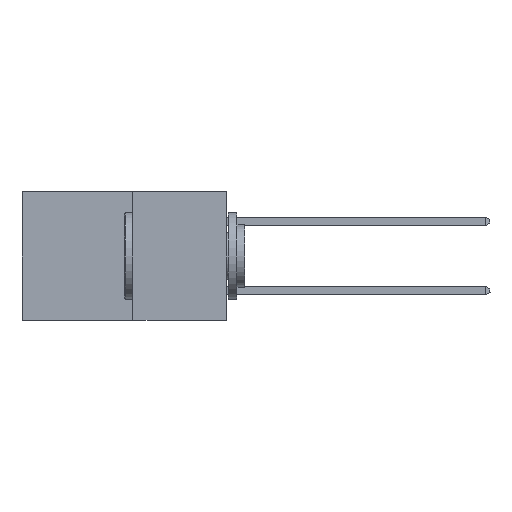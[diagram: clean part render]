
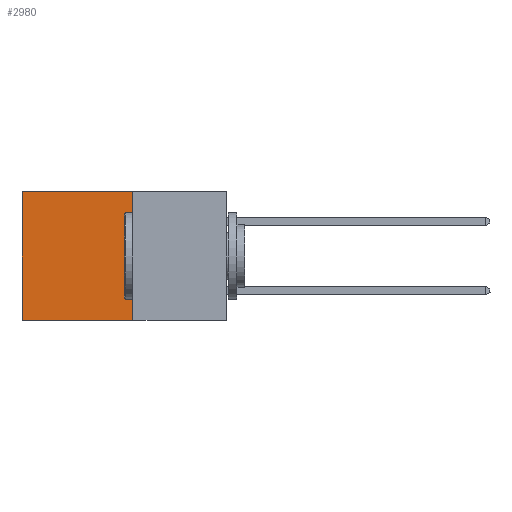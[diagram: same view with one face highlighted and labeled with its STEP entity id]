
A CAD part, left-side view. The second image highlights one B-rep face of the part: STEP entity #2980.
In plain terms, the highlighted planar face has unit normal (-1, 0, 0).
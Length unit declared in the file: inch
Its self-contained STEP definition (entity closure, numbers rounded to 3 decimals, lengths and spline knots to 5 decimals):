
#1551 = LINE ( 'NONE', #14602, #8207 ) ;
#2940 = VECTOR ( 'NONE', #19066, 39.37008 ) ;
#2980 = ADVANCED_FACE ( 'NONE', ( #14730 ), #12413, .F. ) ;
#3741 = EDGE_LOOP ( 'NONE', ( #17220, #11956, #30490, #20516 ) ) ;
#6551 = CARTESIAN_POINT ( 'NONE',  ( 0.277, 0.59, -0.37 ) ) ;
#8207 = VECTOR ( 'NONE', #31452, 39.37008 ) ;
#8642 = CARTESIAN_POINT ( 'NONE',  ( 0.277, 0.27, -0.37 ) ) ;
#9600 = LINE ( 'NONE', #11668, #2940 ) ;
#10718 = VECTOR ( 'NONE', #21757, 39.37008 ) ;
#11668 = CARTESIAN_POINT ( 'NONE',  ( 0.277, 0.27, -0.37 ) ) ;
#11956 = ORIENTED_EDGE ( 'NONE', *, *, #24869, .F. ) ;
#12086 = DIRECTION ( 'NONE',  ( 0., 0., -1. ) ) ;
#12127 = DIRECTION ( 'NONE',  ( 1., 0., 0. ) ) ;
#12413 = PLANE ( 'NONE',  #14323 ) ;
#12559 = CARTESIAN_POINT ( 'NONE',  ( 0.277, 0.27, -0.37 ) ) ;
#13014 = VERTEX_POINT ( 'NONE', #8642 ) ;
#13488 = VECTOR ( 'NONE', #16555, 39.37008 ) ;
#14093 = CARTESIAN_POINT ( 'NONE',  ( 0.277, 0.59, -0.37 ) ) ;
#14323 = AXIS2_PLACEMENT_3D ( 'NONE', #12559, #12127, #12086 ) ;
#14602 = CARTESIAN_POINT ( 'NONE',  ( 0.277, 0.27, 0. ) ) ;
#14627 = EDGE_CURVE ( 'NONE', #21737, #13014, #23674, .T. ) ;
#14730 = FACE_OUTER_BOUND ( 'NONE', #3741, .T. ) ;
#16555 = DIRECTION ( 'NONE',  ( 0., 0., -1. ) ) ;
#17220 = ORIENTED_EDGE ( 'NONE', *, *, #23754, .T. ) ;
#17241 = EDGE_CURVE ( 'NONE', #21737, #30504, #1551, .T. ) ;
#18993 = CARTESIAN_POINT ( 'NONE',  ( 0.277, 0.27, 0. ) ) ;
#19066 = DIRECTION ( 'NONE',  ( 0., 1., 0. ) ) ;
#19327 = CARTESIAN_POINT ( 'NONE',  ( 0.277, 0.27, -0.37 ) ) ;
#19961 = LINE ( 'NONE', #14093, #13488 ) ;
#20516 = ORIENTED_EDGE ( 'NONE', *, *, #17241, .T. ) ;
#20989 = VERTEX_POINT ( 'NONE', #6551 ) ;
#21737 = VERTEX_POINT ( 'NONE', #18993 ) ;
#21757 = DIRECTION ( 'NONE',  ( 0., 0., -1. ) ) ;
#23674 = LINE ( 'NONE', #19327, #10718 ) ;
#23754 = EDGE_CURVE ( 'NONE', #30504, #20989, #19961, .T. ) ;
#24869 = EDGE_CURVE ( 'NONE', #13014, #20989, #9600, .T. ) ;
#26931 = CARTESIAN_POINT ( 'NONE',  ( 0.277, 0.59, 0. ) ) ;
#30490 = ORIENTED_EDGE ( 'NONE', *, *, #14627, .F. ) ;
#30504 = VERTEX_POINT ( 'NONE', #26931 ) ;
#31452 = DIRECTION ( 'NONE',  ( 0., 1., 0. ) ) ;
